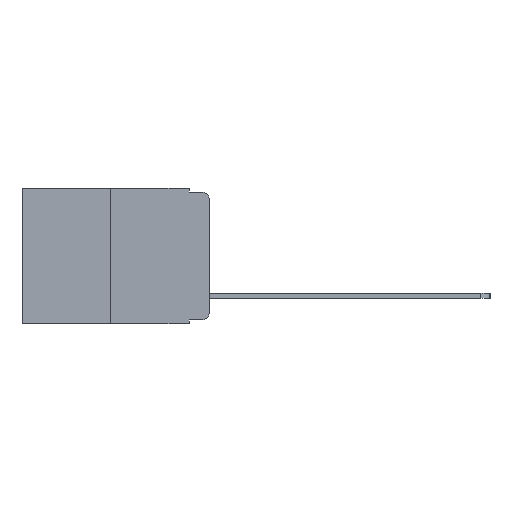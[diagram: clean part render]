
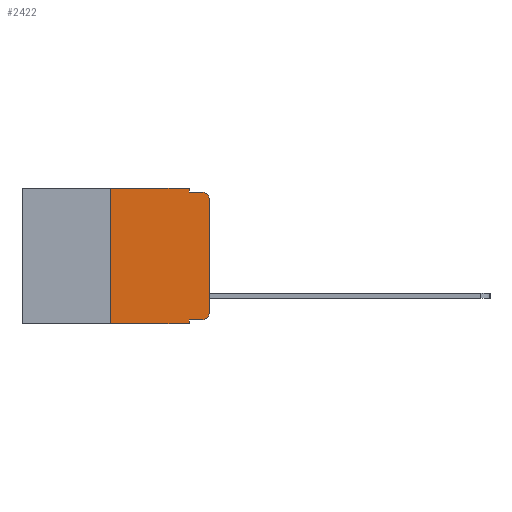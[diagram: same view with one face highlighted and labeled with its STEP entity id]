
A CAD part, left-side view. The second image highlights one B-rep face of the part: STEP entity #2422.
In plain terms, the highlighted planar face has unit normal (-1, 0, 0).
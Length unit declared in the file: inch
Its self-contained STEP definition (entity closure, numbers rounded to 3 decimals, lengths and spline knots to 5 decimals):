
#332 = VERTEX_POINT ( 'NONE', #2634 ) ;
#354 = DIRECTION ( 'NONE',  ( 0., -1., 0. ) ) ;
#647 = VERTEX_POINT ( 'NONE', #2202 ) ;
#658 = EDGE_CURVE ( 'NONE', #647, #6982, #6220, .T. ) ;
#700 = DIRECTION ( 'NONE',  ( -1., 0., 0. ) ) ;
#812 = EDGE_CURVE ( 'NONE', #8935, #332, #10584, .T. ) ;
#872 = AXIS2_PLACEMENT_3D ( 'NONE', #6553, #700, #7450 ) ;
#958 = CARTESIAN_POINT ( 'NONE',  ( 0., 0.473, 0. ) ) ;
#1242 = EDGE_LOOP ( 'NONE', ( #3326, #3189, #9722, #5422, #5678, #7716, #10220, #10210, #10457, #5934 ) ) ;
#1250 = CARTESIAN_POINT ( 'NONE',  ( 0., 0.02, -0.01 ) ) ;
#1478 = EDGE_CURVE ( 'NONE', #6982, #10162, #4427, .T. ) ;
#1527 = CARTESIAN_POINT ( 'NONE',  ( 0., 0.25, -0.343 ) ) ;
#1717 = EDGE_CURVE ( 'NONE', #647, #1732, #4712, .T. ) ;
#1732 = VERTEX_POINT ( 'NONE', #11668 ) ;
#1911 = FACE_OUTER_BOUND ( 'NONE', #1242, .T. ) ;
#1913 = LINE ( 'NONE', #5830, #6673 ) ;
#2202 = CARTESIAN_POINT ( 'NONE',  ( 0., 0.051, -0.333 ) ) ;
#2226 = CARTESIAN_POINT ( 'NONE',  ( 0., 0., -0.313 ) ) ;
#2422 = ADVANCED_FACE ( 'NONE', ( #1911 ), #5071, .F. ) ;
#2634 = CARTESIAN_POINT ( 'NONE',  ( 0., 0.051, 0. ) ) ;
#2747 = EDGE_CURVE ( 'NONE', #332, #6227, #1913, .T. ) ;
#2764 = EDGE_CURVE ( 'NONE', #4759, #8935, #4350, .T. ) ;
#2885 = CARTESIAN_POINT ( 'NONE',  ( 0., 0., -0.03 ) ) ;
#3011 = CIRCLE ( 'NONE', #872, 0.02 ) ;
#3180 = EDGE_CURVE ( 'NONE', #6227, #3729, #5337, .T. ) ;
#3189 = ORIENTED_EDGE ( 'NONE', *, *, #6115, .T. ) ;
#3326 = ORIENTED_EDGE ( 'NONE', *, *, #6972, .T. ) ;
#3369 = CARTESIAN_POINT ( 'NONE',  ( 0., 0.02, -0.313 ) ) ;
#3652 = CARTESIAN_POINT ( 'NONE',  ( 0., 0.051, -0.333 ) ) ;
#3729 = VERTEX_POINT ( 'NONE', #1250 ) ;
#3781 = VECTOR ( 'NONE', #6969, 39.37008 ) ;
#3847 = VECTOR ( 'NONE', #354, 39.37008 ) ;
#4250 = VECTOR ( 'NONE', #11391, 39.37008 ) ;
#4289 = CARTESIAN_POINT ( 'NONE',  ( 0., 0.051, -0.01 ) ) ;
#4350 = LINE ( 'NONE', #8511, #6393 ) ;
#4427 = CIRCLE ( 'NONE', #11096, 0.02 ) ;
#4712 = LINE ( 'NONE', #7000, #7016 ) ;
#4759 = VERTEX_POINT ( 'NONE', #1527 ) ;
#5071 = PLANE ( 'NONE',  #11339 ) ;
#5245 = CARTESIAN_POINT ( 'NONE',  ( 0., 0., 0. ) ) ;
#5337 = LINE ( 'NONE', #4289, #8569 ) ;
#5422 = ORIENTED_EDGE ( 'NONE', *, *, #2747, .F. ) ;
#5678 = ORIENTED_EDGE ( 'NONE', *, *, #812, .F. ) ;
#5800 = CARTESIAN_POINT ( 'NONE',  ( 0., 0.051, -0.01 ) ) ;
#5830 = CARTESIAN_POINT ( 'NONE',  ( 0., 0.051, 0. ) ) ;
#5868 = DIRECTION ( 'NONE',  ( 0., 0., -1. ) ) ;
#5925 = DIRECTION ( 'NONE',  ( 0., 0., -1. ) ) ;
#5934 = ORIENTED_EDGE ( 'NONE', *, *, #1478, .T. ) ;
#6092 = VECTOR ( 'NONE', #9182, 39.37008 ) ;
#6115 = EDGE_CURVE ( 'NONE', #6141, #3729, #3011, .T. ) ;
#6141 = VERTEX_POINT ( 'NONE', #2885 ) ;
#6173 = LINE ( 'NONE', #5245, #3781 ) ;
#6220 = LINE ( 'NONE', #3652, #3847 ) ;
#6227 = VERTEX_POINT ( 'NONE', #5800 ) ;
#6301 = LINE ( 'NONE', #8137, #4250 ) ;
#6393 = VECTOR ( 'NONE', #10933, 39.37008 ) ;
#6395 = DIRECTION ( 'NONE',  ( 0., 0., -1. ) ) ;
#6490 = DIRECTION ( 'NONE',  ( 0., 0., -1. ) ) ;
#6553 = CARTESIAN_POINT ( 'NONE',  ( 0., 0.02, -0.03 ) ) ;
#6673 = VECTOR ( 'NONE', #5868, 39.37008 ) ;
#6969 = DIRECTION ( 'NONE',  ( 0., 0., 1. ) ) ;
#6972 = EDGE_CURVE ( 'NONE', #10162, #6141, #6173, .T. ) ;
#6982 = VERTEX_POINT ( 'NONE', #8700 ) ;
#7000 = CARTESIAN_POINT ( 'NONE',  ( 0., 0.051, 0. ) ) ;
#7016 = VECTOR ( 'NONE', #6395, 39.37008 ) ;
#7450 = DIRECTION ( 'NONE',  ( 0., 0., -1. ) ) ;
#7716 = ORIENTED_EDGE ( 'NONE', *, *, #2764, .F. ) ;
#7812 = DIRECTION ( 'NONE',  ( 0., -1., 0. ) ) ;
#7853 = CARTESIAN_POINT ( 'NONE',  ( 0., 0.25, 0. ) ) ;
#8137 = CARTESIAN_POINT ( 'NONE',  ( 0., 0.473, -0.343 ) ) ;
#8511 = CARTESIAN_POINT ( 'NONE',  ( 0., 0.25, 0. ) ) ;
#8569 = VECTOR ( 'NONE', #7812, 39.37008 ) ;
#8639 = DIRECTION ( 'NONE',  ( -1., 0., 0. ) ) ;
#8700 = CARTESIAN_POINT ( 'NONE',  ( 0., 0.02, -0.333 ) ) ;
#8935 = VERTEX_POINT ( 'NONE', #7853 ) ;
#9182 = DIRECTION ( 'NONE',  ( 0., -1., 0. ) ) ;
#9683 = CARTESIAN_POINT ( 'NONE',  ( 0., 0.473, 0. ) ) ;
#9722 = ORIENTED_EDGE ( 'NONE', *, *, #3180, .F. ) ;
#10162 = VERTEX_POINT ( 'NONE', #2226 ) ;
#10210 = ORIENTED_EDGE ( 'NONE', *, *, #1717, .F. ) ;
#10220 = ORIENTED_EDGE ( 'NONE', *, *, #10628, .T. ) ;
#10457 = ORIENTED_EDGE ( 'NONE', *, *, #658, .T. ) ;
#10584 = LINE ( 'NONE', #9683, #6092 ) ;
#10628 = EDGE_CURVE ( 'NONE', #4759, #1732, #6301, .T. ) ;
#10933 = DIRECTION ( 'NONE',  ( 0., 0., 1. ) ) ;
#10980 = DIRECTION ( 'NONE',  ( 1., 0., 0. ) ) ;
#11096 = AXIS2_PLACEMENT_3D ( 'NONE', #3369, #8639, #6490 ) ;
#11339 = AXIS2_PLACEMENT_3D ( 'NONE', #958, #10980, #5925 ) ;
#11391 = DIRECTION ( 'NONE',  ( 0., -1., 0. ) ) ;
#11668 = CARTESIAN_POINT ( 'NONE',  ( 0., 0.051, -0.343 ) ) ;
